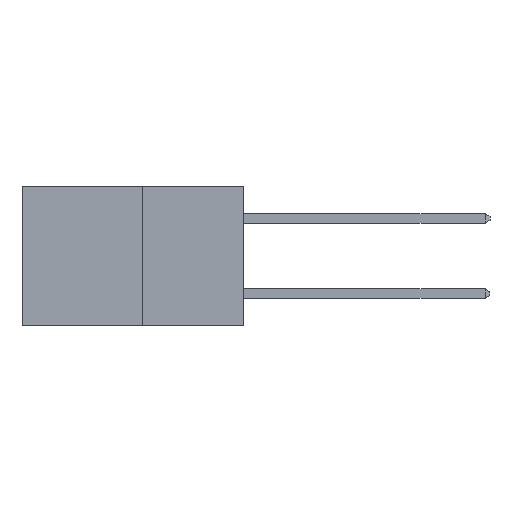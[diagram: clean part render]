
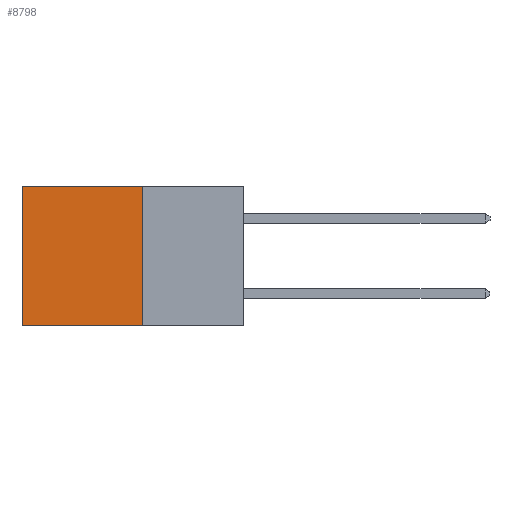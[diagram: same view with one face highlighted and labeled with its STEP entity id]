
A CAD part, left-side view. The second image highlights one B-rep face of the part: STEP entity #8798.
In plain terms, the highlighted planar face has unit normal (-1, 0, 0).
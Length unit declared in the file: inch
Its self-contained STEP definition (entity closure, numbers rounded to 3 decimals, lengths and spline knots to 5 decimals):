
#464 = PLANE ( 'NONE',  #7728 ) ;
#555 = LINE ( 'NONE', #1939, #4435 ) ;
#1178 = VECTOR ( 'NONE', #7117, 39.37008 ) ;
#1319 = CARTESIAN_POINT ( 'NONE',  ( 0.277, 0.27, -0.37 ) ) ;
#1361 = VECTOR ( 'NONE', #2338, 39.37008 ) ;
#1386 = CARTESIAN_POINT ( 'NONE',  ( 0.277, 0.27, 0. ) ) ;
#1474 = EDGE_LOOP ( 'NONE', ( #4715, #2807, #4371, #6037 ) ) ;
#1755 = CARTESIAN_POINT ( 'NONE',  ( 0.277, 0.27, 0. ) ) ;
#1939 = CARTESIAN_POINT ( 'NONE',  ( 0.277, 0.27, -0.37 ) ) ;
#1968 = DIRECTION ( 'NONE',  ( 1., 0., 0. ) ) ;
#2338 = DIRECTION ( 'NONE',  ( 0., 0., -1. ) ) ;
#2388 = CARTESIAN_POINT ( 'NONE',  ( 0.277, 0.59, -0.37 ) ) ;
#2413 = VECTOR ( 'NONE', #7682, 39.37008 ) ;
#2807 = ORIENTED_EDGE ( 'NONE', *, *, #4655, .F. ) ;
#4117 = EDGE_CURVE ( 'NONE', #6004, #4497, #8394, .T. ) ;
#4312 = FACE_OUTER_BOUND ( 'NONE', #1474, .T. ) ;
#4371 = ORIENTED_EDGE ( 'NONE', *, *, #7040, .F. ) ;
#4435 = VECTOR ( 'NONE', #5494, 39.37008 ) ;
#4497 = VERTEX_POINT ( 'NONE', #8260 ) ;
#4655 = EDGE_CURVE ( 'NONE', #8352, #4830, #7972, .T. ) ;
#4715 = ORIENTED_EDGE ( 'NONE', *, *, #5899, .T. ) ;
#4830 = VERTEX_POINT ( 'NONE', #6803 ) ;
#5494 = DIRECTION ( 'NONE',  ( 0., 0., -1. ) ) ;
#5899 = EDGE_CURVE ( 'NONE', #4497, #4830, #8754, .T. ) ;
#6004 = VERTEX_POINT ( 'NONE', #1755 ) ;
#6037 = ORIENTED_EDGE ( 'NONE', *, *, #4117, .T. ) ;
#6212 = CARTESIAN_POINT ( 'NONE',  ( 0.277, 0.27, -0.37 ) ) ;
#6803 = CARTESIAN_POINT ( 'NONE',  ( 0.277, 0.59, -0.37 ) ) ;
#6881 = DIRECTION ( 'NONE',  ( 0., 0., -1. ) ) ;
#7040 = EDGE_CURVE ( 'NONE', #6004, #8352, #555, .T. ) ;
#7117 = DIRECTION ( 'NONE',  ( 0., 1., 0. ) ) ;
#7658 = CARTESIAN_POINT ( 'NONE',  ( 0.277, 0.27, -0.37 ) ) ;
#7682 = DIRECTION ( 'NONE',  ( 0., 1., 0. ) ) ;
#7728 = AXIS2_PLACEMENT_3D ( 'NONE', #6212, #1968, #6881 ) ;
#7972 = LINE ( 'NONE', #7658, #2413 ) ;
#8260 = CARTESIAN_POINT ( 'NONE',  ( 0.277, 0.59, 0. ) ) ;
#8352 = VERTEX_POINT ( 'NONE', #1319 ) ;
#8394 = LINE ( 'NONE', #1386, #1178 ) ;
#8754 = LINE ( 'NONE', #2388, #1361 ) ;
#8798 = ADVANCED_FACE ( 'NONE', ( #4312 ), #464, .F. ) ;
